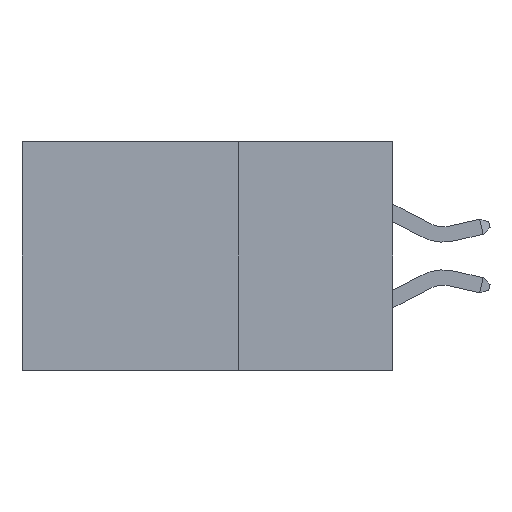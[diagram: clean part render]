
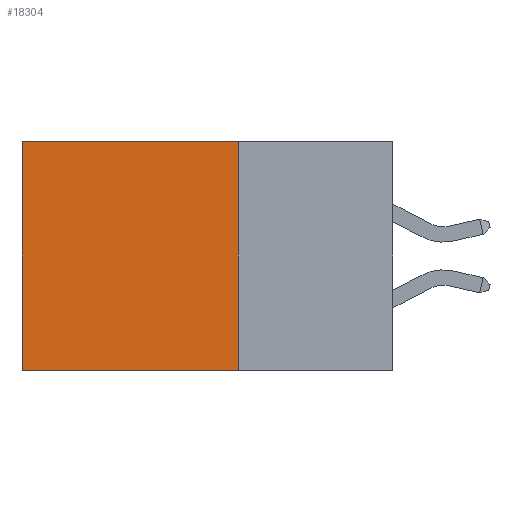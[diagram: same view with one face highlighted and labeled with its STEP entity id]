
A CAD part, left-side view. The second image highlights one B-rep face of the part: STEP entity #18304.
In plain terms, the highlighted planar face has unit normal (-1, 0, 0).
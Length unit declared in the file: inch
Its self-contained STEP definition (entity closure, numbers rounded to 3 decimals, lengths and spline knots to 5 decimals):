
#1514 = EDGE_CURVE ( 'NONE', #25631, #15612, #33370, .T. ) ;
#1882 = EDGE_CURVE ( 'NONE', #25631, #19017, #15161, .T. ) ;
#4517 = CARTESIAN_POINT ( 'NONE',  ( 0.2875, 0.6, 0. ) ) ;
#4604 = EDGE_CURVE ( 'NONE', #19017, #33538, #29606, .T. ) ;
#5760 = VECTOR ( 'NONE', #29331, 39.37008 ) ;
#6627 = PLANE ( 'NONE',  #31665 ) ;
#7670 = ORIENTED_EDGE ( 'NONE', *, *, #12814, .F. ) ;
#9395 = DIRECTION ( 'NONE',  ( 1., 0., 0. ) ) ;
#9558 = ORIENTED_EDGE ( 'NONE', *, *, #1514, .F. ) ;
#9714 = CARTESIAN_POINT ( 'NONE',  ( 0.2875, 0.25, -0.37 ) ) ;
#10378 = ORIENTED_EDGE ( 'NONE', *, *, #1882, .T. ) ;
#11142 = CARTESIAN_POINT ( 'NONE',  ( 0.2875, 0.25, 0. ) ) ;
#12814 = EDGE_CURVE ( 'NONE', #15612, #33538, #26038, .T. ) ;
#13180 = CARTESIAN_POINT ( 'NONE',  ( 0.2875, 0.25, 0. ) ) ;
#13264 = CARTESIAN_POINT ( 'NONE',  ( 0.2875, 0.25, -0.37 ) ) ;
#15109 = DIRECTION ( 'NONE',  ( 0., 1., 0. ) ) ;
#15161 = LINE ( 'NONE', #17741, #28195 ) ;
#15612 = VERTEX_POINT ( 'NONE', #9714 ) ;
#16222 = CARTESIAN_POINT ( 'NONE',  ( 0.2875, 0.6, 0. ) ) ;
#16266 = FACE_OUTER_BOUND ( 'NONE', #24556, .T. ) ;
#17741 = CARTESIAN_POINT ( 'NONE',  ( 0.2875, 0.25, 0. ) ) ;
#18304 = ADVANCED_FACE ( 'NONE', ( #16266 ), #6627, .F. ) ;
#18565 = DIRECTION ( 'NONE',  ( 0., 1., 0. ) ) ;
#19017 = VERTEX_POINT ( 'NONE', #4517 ) ;
#21487 = DIRECTION ( 'NONE',  ( 0., 0., -1. ) ) ;
#22748 = VECTOR ( 'NONE', #21487, 39.37008 ) ;
#24556 = EDGE_LOOP ( 'NONE', ( #30658, #7670, #9558, #10378 ) ) ;
#25020 = CARTESIAN_POINT ( 'NONE',  ( 0.2875, 0.25, 0. ) ) ;
#25631 = VERTEX_POINT ( 'NONE', #13180 ) ;
#26038 = LINE ( 'NONE', #13264, #26389 ) ;
#26389 = VECTOR ( 'NONE', #18565, 39.37008 ) ;
#27638 = DIRECTION ( 'NONE',  ( 0., 0., -1. ) ) ;
#27936 = CARTESIAN_POINT ( 'NONE',  ( 0.2875, 0.6, -0.37 ) ) ;
#28195 = VECTOR ( 'NONE', #15109, 39.37008 ) ;
#29331 = DIRECTION ( 'NONE',  ( 0., 0., -1. ) ) ;
#29606 = LINE ( 'NONE', #16222, #22748 ) ;
#30658 = ORIENTED_EDGE ( 'NONE', *, *, #4604, .T. ) ;
#31665 = AXIS2_PLACEMENT_3D ( 'NONE', #25020, #9395, #27638 ) ;
#33370 = LINE ( 'NONE', #11142, #5760 ) ;
#33538 = VERTEX_POINT ( 'NONE', #27936 ) ;
